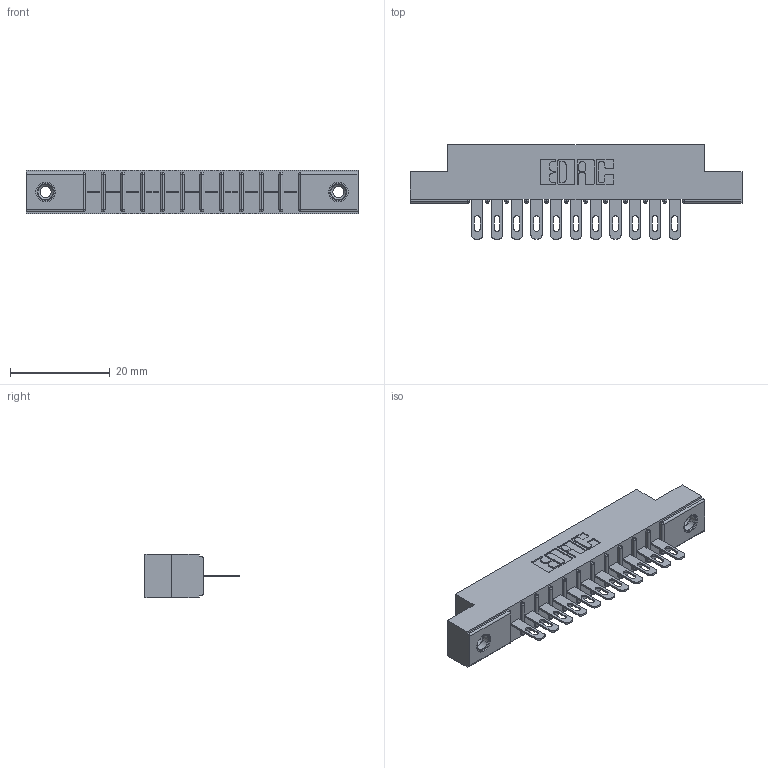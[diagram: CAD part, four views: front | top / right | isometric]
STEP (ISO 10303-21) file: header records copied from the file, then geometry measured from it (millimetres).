
FILE_DESCRIPTION (( 'STEP AP203' ), '1' );
FILE_NAME ('356-011-500-108.STEP', '2018-07-31T07:09:25', ( '' ), ( '' ), 'SwSTEP 2.0', 'SolidWorks 2016', '' );
FILE_SCHEMA (( 'CONFIG_CONTROL_DESIGN' ));
Length unit declared in the file: inch
Products named in the file (4): 345-250-001_345-250-003-102; 356-011-500-108; 306 Part_.156 Dia; 306-290-001_100
Assembly tree (14 placements, depth 2):
  356-011-500-108
    306 Part_.156 Dia
    306-290-001_100  x11
    345-250-001_345-250-003-102  x2
Bounding box: 66.6 x 18.87 x 8.71 mm (x, y, z)
Volume: 4531.2 mm3; surface area: 6561.9 mm2
Topology: 14 solids, 14 shells, 1012 faces, 2817 edges, 1810 vertices
Faces by surface type: plane 650, cylinder 302, sphere 44, cone 12, torus 4
Entity records: 15623 total; most frequent: CARTESIAN_POINT 2599, DIRECTION 2575, ORIENTED_EDGE 2566, EDGE_CURVE 1283, LINE 983, VECTOR 983, VERTEX_POINT 820, AXIS2_PLACEMENT_3D 796
